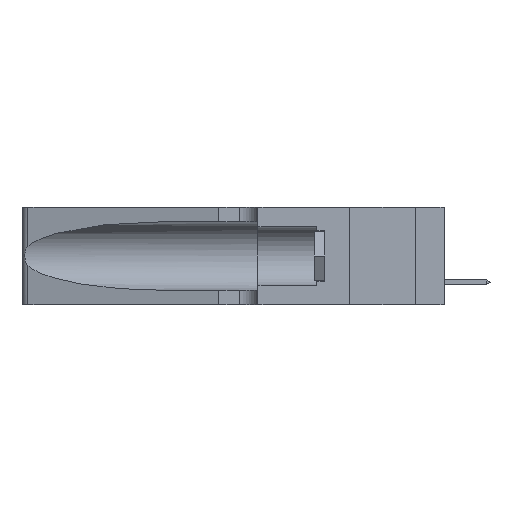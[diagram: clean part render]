
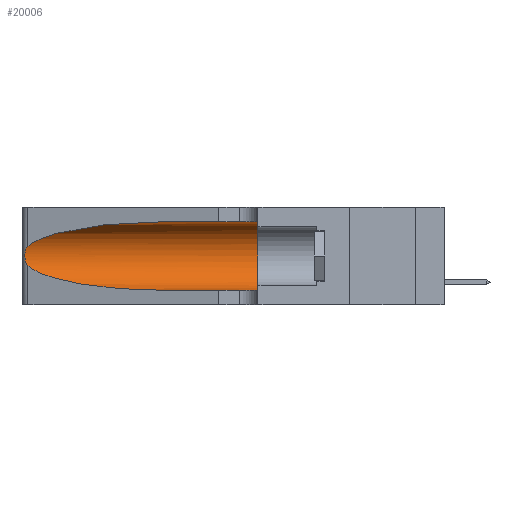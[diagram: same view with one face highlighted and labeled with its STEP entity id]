
A CAD part, left-side view. The second image highlights one B-rep face of the part: STEP entity #20006.
In plain terms, the highlighted cylindrical face has radius 3.308 mm (diameter 6.617 mm), a partial arc.
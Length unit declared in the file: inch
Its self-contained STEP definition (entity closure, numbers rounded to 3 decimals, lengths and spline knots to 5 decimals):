
#27 = CARTESIAN_POINT ( 'NONE',  ( 0.1305, 0.72297, 0.05475 ) ) ;
#98 = VERTEX_POINT ( 'NONE', #9790 ) ;
#136 = CARTESIAN_POINT ( 'NONE',  ( 0.1305, 1.61858, 0.05475 ) ) ;
#875 = CARTESIAN_POINT ( 'NONE',  ( 0.1305, 1.61858, 0.31525 ) ) ;
#1018 = CARTESIAN_POINT ( 'NONE',  ( 0.1305, 0.72297, 0.31525 ) ) ;
#1154 = EDGE_CURVE ( 'NONE', #14808, #10334, #20559, .T. ) ;
#2254 = DIRECTION ( 'NONE',  ( 0., -1., 0. ) ) ;
#3176 = CARTESIAN_POINT ( 'NONE',  ( 0.25487, 1.22718, 0.22369 ) ) ;
#3282 = AXIS2_PLACEMENT_3D ( 'NONE', #7673, #2254, #17530 ) ;
#4117 = CYLINDRICAL_SURFACE ( 'NONE', #3282, 0.13025 ) ;
#4385 = CARTESIAN_POINT ( 'NONE',  ( 0.1305, 0.35, 0.185 ) ) ;
#4486 = EDGE_CURVE ( 'NONE', #12038, #10334, #5710, .T. ) ;
#4884 = ORIENTED_EDGE ( 'NONE', *, *, #1154, .F. ) ;
#5312 = ORIENTED_EDGE ( 'NONE', *, *, #23765, .T. ) ;
#5710 = LINE ( 'NONE', #136, #17683 ) ;
#5811 = ORIENTED_EDGE ( 'NONE', *, *, #24058, .F. ) ;
#5939 = ORIENTED_EDGE ( 'NONE', *, *, #24759, .T. ) ;
#6836 =( BOUNDED_CURVE ( )  B_SPLINE_CURVE ( 3, ( #21051, #19031, #15129, #18950 ),
 .UNSPECIFIED., .F., .F. ) 
 B_SPLINE_CURVE_WITH_KNOTS ( ( 4, 4 ),
 ( 3.44316, 4.71239 ),
 .UNSPECIFIED. ) 
 CURVE ( )  GEOMETRIC_REPRESENTATION_ITEM ( )  RATIONAL_B_SPLINE_CURVE ( ( 1., 0.87, 0.87, 1. ) ) 
 REPRESENTATION_ITEM ( '' )  );
#6896 = DIRECTION ( 'NONE',  ( 0., -1., 0. ) ) ;
#6953 = CARTESIAN_POINT ( 'NONE',  ( 0.25856, 1.23593, 0.16098 ) ) ;
#7024 = CARTESIAN_POINT ( 'NONE',  ( 0.25787, 1.23484, 0.2124 ) ) ;
#7673 = CARTESIAN_POINT ( 'NONE',  ( 0.1305, 1.61858, 0.185 ) ) ;
#8867 = CARTESIAN_POINT ( 'NONE',  ( 0.25639, 1.23186, 0.15144 ) ) ;
#9790 = CARTESIAN_POINT ( 'NONE',  ( 0.25487, 1.22718, 0.22369 ) ) ;
#10053 = CARTESIAN_POINT ( 'NONE',  ( 0.1305, 0.35, 0.31525 ) ) ;
#10334 = VERTEX_POINT ( 'NONE', #15677 ) ;
#10875 = CARTESIAN_POINT ( 'NONE',  ( 0.25555, 1.22993, 0.14849 ) ) ;
#12038 = VERTEX_POINT ( 'NONE', #27 ) ;
#12460 = CARTESIAN_POINT ( 'NONE',  ( 0.25789, 1.23486, 0.15765 ) ) ;
#12796 = CARTESIAN_POINT ( 'NONE',  ( 0.26017, 1.23833, 0.17102 ) ) ;
#14013 = DIRECTION ( 'NONE',  ( 0., 0., 1. ) ) ;
#14409 = CARTESIAN_POINT ( 'NONE',  ( 0.2373, 1.15595, 0.28018 ) ) ;
#14496 = CARTESIAN_POINT ( 'NONE',  ( 0.26075, 1.23896, 0.19203 ) ) ;
#14808 = VERTEX_POINT ( 'NONE', #10053 ) ;
#14950 =( BOUNDED_CURVE ( )  B_SPLINE_CURVE ( 3, ( #1018, #18810, #14409, #16981 ),
 .UNSPECIFIED., .F., .T. ) 
 B_SPLINE_CURVE_WITH_KNOTS ( ( 4, 4 ),
 ( 1.5708, 2.84003 ),
 .UNSPECIFIED. ) 
 CURVE ( )  GEOMETRIC_REPRESENTATION_ITEM ( )  RATIONAL_B_SPLINE_CURVE ( ( 1., 0.87, 0.87, 1. ) ) 
 REPRESENTATION_ITEM ( '' )  );
#15129 = CARTESIAN_POINT ( 'NONE',  ( 0.18966, 0.96281, 0.05475 ) ) ;
#15317 = VECTOR ( 'NONE', #6896, 39.37008 ) ;
#15677 = CARTESIAN_POINT ( 'NONE',  ( 0.1305, 0.35, 0.05475 ) ) ;
#16255 = VERTEX_POINT ( 'NONE', #23937 ) ;
#16501 = B_SPLINE_CURVE_WITH_KNOTS ( 'NONE', 3,
 ( #3176, #20251, #16572, #7024, #22172, #22334, #14496, #23906, #12796, #6953, #12460, #8867, #10875, #24232 ),
 .UNSPECIFIED., .F., .F.,
 ( 4, 2, 2, 2, 2, 2, 4 ),
 ( 0., 0.00027, 0.00053, 0.00107, 0.0016, 0.00187, 0.00214 ),
 .UNSPECIFIED. ) ;
#16572 = CARTESIAN_POINT ( 'NONE',  ( 0.25639, 1.23184, 0.21858 ) ) ;
#16696 = FACE_OUTER_BOUND ( 'NONE', #23011, .T. ) ;
#16981 = CARTESIAN_POINT ( 'NONE',  ( 0.25487, 1.22718, 0.22369 ) ) ;
#17332 = DIRECTION ( 'NONE',  ( 0., -1., 0. ) ) ;
#17501 = DIRECTION ( 'NONE',  ( 0., 1., 0. ) ) ;
#17530 = DIRECTION ( 'NONE',  ( 0., 0., -1. ) ) ;
#17581 = CARTESIAN_POINT ( 'NONE',  ( 0.25487, 1.22718, 0.14631 ) ) ;
#17683 = VECTOR ( 'NONE', #17332, 39.37008 ) ;
#18290 = ORIENTED_EDGE ( 'NONE', *, *, #4486, .T. ) ;
#18810 = CARTESIAN_POINT ( 'NONE',  ( 0.18966, 0.96281, 0.31525 ) ) ;
#18950 = CARTESIAN_POINT ( 'NONE',  ( 0.1305, 0.72297, 0.05475 ) ) ;
#19031 = CARTESIAN_POINT ( 'NONE',  ( 0.2373, 1.15595, 0.08982 ) ) ;
#19667 = VERTEX_POINT ( 'NONE', #17581 ) ;
#20006 = ADVANCED_FACE ( 'NONE', ( #16696 ), #4117, .F. ) ;
#20251 = CARTESIAN_POINT ( 'NONE',  ( 0.25555, 1.22994, 0.2215 ) ) ;
#20559 = CIRCLE ( 'NONE', #23914, 0.13025 ) ;
#20634 = EDGE_CURVE ( 'NONE', #16255, #98, #14950, .T. ) ;
#21051 = CARTESIAN_POINT ( 'NONE',  ( 0.25487, 1.22718, 0.14631 ) ) ;
#22172 = CARTESIAN_POINT ( 'NONE',  ( 0.25854, 1.2359, 0.20912 ) ) ;
#22334 = CARTESIAN_POINT ( 'NONE',  ( 0.26018, 1.23835, 0.19895 ) ) ;
#23011 = EDGE_LOOP ( 'NONE', ( #23095, #5939, #5312, #18290, #4884, #5811 ) ) ;
#23018 = LINE ( 'NONE', #875, #15317 ) ;
#23095 = ORIENTED_EDGE ( 'NONE', *, *, #20634, .T. ) ;
#23765 = EDGE_CURVE ( 'NONE', #19667, #12038, #6836, .T. ) ;
#23906 = CARTESIAN_POINT ( 'NONE',  ( 0.26075, 1.23896, 0.178 ) ) ;
#23914 = AXIS2_PLACEMENT_3D ( 'NONE', #4385, #17501, #14013 ) ;
#23937 = CARTESIAN_POINT ( 'NONE',  ( 0.1305, 0.72297, 0.31525 ) ) ;
#24058 = EDGE_CURVE ( 'NONE', #16255, #14808, #23018, .T. ) ;
#24232 = CARTESIAN_POINT ( 'NONE',  ( 0.25487, 1.22718, 0.14631 ) ) ;
#24759 = EDGE_CURVE ( 'NONE', #98, #19667, #16501, .T. ) ;
